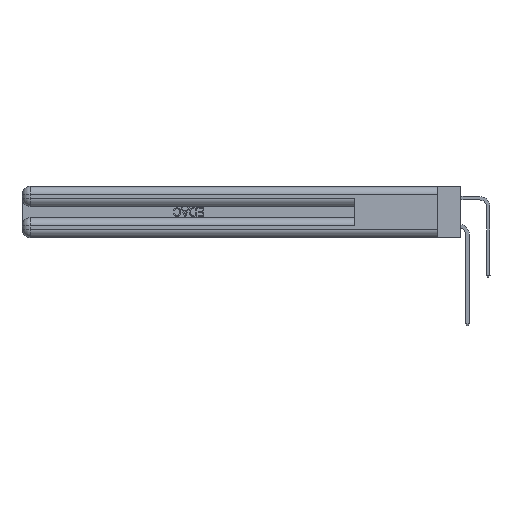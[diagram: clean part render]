
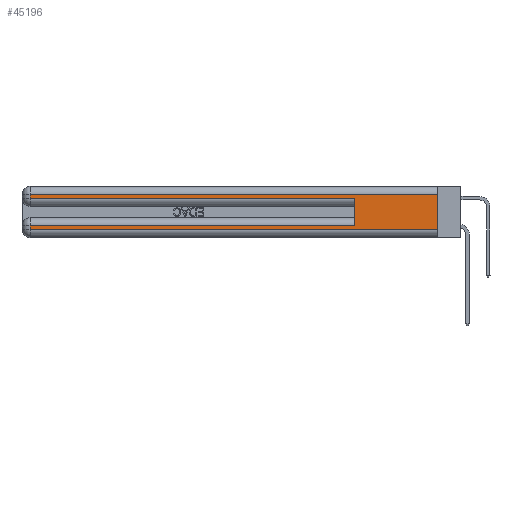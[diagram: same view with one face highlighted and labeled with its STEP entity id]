
A CAD part, left-side view. The second image highlights one B-rep face of the part: STEP entity #45196.
In plain terms, the highlighted planar face has unit normal (-1, 0, 0).
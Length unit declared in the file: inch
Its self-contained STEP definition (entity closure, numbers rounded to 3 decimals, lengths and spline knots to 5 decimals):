
#705 = DIRECTION ( 'NONE',  ( 0., 0., -1. ) ) ;
#1729 = EDGE_LOOP ( 'NONE', ( #14776, #45961, #12684, #37236, #11976, #14277, #4762, #40636 ) ) ;
#2583 = CARTESIAN_POINT ( 'NONE',  ( 0., 0., 0.06 ) ) ;
#3028 = CARTESIAN_POINT ( 'NONE',  ( 0., 0., 0.085 ) ) ;
#3943 = CARTESIAN_POINT ( 'NONE',  ( 0., 0.6, 0.145 ) ) ;
#4076 = CARTESIAN_POINT ( 'NONE',  ( 0., 0., 0.37 ) ) ;
#4349 = CARTESIAN_POINT ( 'NONE',  ( 0., 0., 0.285 ) ) ;
#4762 = ORIENTED_EDGE ( 'NONE', *, *, #11932, .T. ) ;
#5708 = EDGE_CURVE ( 'NONE', #19488, #32382, #12254, .T. ) ;
#5783 = CARTESIAN_POINT ( 'NONE',  ( 0., 0.6, 0.285 ) ) ;
#6198 = CARTESIAN_POINT ( 'NONE',  ( 0., 0.6, 0.085 ) ) ;
#6210 = VERTEX_POINT ( 'NONE', #19392 ) ;
#6652 = LINE ( 'NONE', #2583, #27688 ) ;
#6951 = CARTESIAN_POINT ( 'NONE',  ( 0., 0., 0.31 ) ) ;
#7152 = EDGE_CURVE ( 'NONE', #19488, #37345, #27515, .T. ) ;
#9133 = LINE ( 'NONE', #25689, #40958 ) ;
#9189 = CARTESIAN_POINT ( 'NONE',  ( 0., 2.94, 0.085 ) ) ;
#11681 = CARTESIAN_POINT ( 'NONE',  ( 0., 0., 0.06 ) ) ;
#11932 = EDGE_CURVE ( 'NONE', #27845, #13278, #39728, .T. ) ;
#11976 = ORIENTED_EDGE ( 'NONE', *, *, #37892, .F. ) ;
#12254 = LINE ( 'NONE', #14886, #40137 ) ;
#12684 = ORIENTED_EDGE ( 'NONE', *, *, #36053, .T. ) ;
#12790 = EDGE_CURVE ( 'NONE', #6210, #20750, #14136, .T. ) ;
#13278 = VERTEX_POINT ( 'NONE', #30140 ) ;
#14136 = LINE ( 'NONE', #4349, #43670 ) ;
#14277 = ORIENTED_EDGE ( 'NONE', *, *, #26749, .T. ) ;
#14776 = ORIENTED_EDGE ( 'NONE', *, *, #7152, .F. ) ;
#14886 = CARTESIAN_POINT ( 'NONE',  ( 0., 0., 0.31 ) ) ;
#16128 = DIRECTION ( 'NONE',  ( 0., -1., 0. ) ) ;
#17498 = DIRECTION ( 'NONE',  ( 0., 0., -1. ) ) ;
#18130 = CARTESIAN_POINT ( 'NONE',  ( 0., 2.94, 0.37 ) ) ;
#19392 = CARTESIAN_POINT ( 'NONE',  ( 0., 2.94, 0.285 ) ) ;
#19488 = VERTEX_POINT ( 'NONE', #6951 ) ;
#20701 = VECTOR ( 'NONE', #45680, 39.37008 ) ;
#20750 = VERTEX_POINT ( 'NONE', #5783 ) ;
#20902 = EDGE_CURVE ( 'NONE', #13278, #37345, #6652, .T. ) ;
#20932 = DIRECTION ( 'NONE',  ( 0., -1., 0. ) ) ;
#22026 = LINE ( 'NONE', #3028, #23170 ) ;
#23170 = VECTOR ( 'NONE', #25055, 39.37008 ) ;
#24401 = VECTOR ( 'NONE', #17498, 39.37008 ) ;
#25055 = DIRECTION ( 'NONE',  ( 0., 1., 0. ) ) ;
#25689 = CARTESIAN_POINT ( 'NONE',  ( 0., 2.94, 0.37 ) ) ;
#26053 = DIRECTION ( 'NONE',  ( 1., 0., 0. ) ) ;
#26078 = DIRECTION ( 'NONE',  ( 0., 0., 1. ) ) ;
#26749 = EDGE_CURVE ( 'NONE', #32132, #27845, #22026, .T. ) ;
#27515 = LINE ( 'NONE', #34404, #20701 ) ;
#27688 = VECTOR ( 'NONE', #20932, 39.37008 ) ;
#27845 = VERTEX_POINT ( 'NONE', #9189 ) ;
#29171 = FACE_OUTER_BOUND ( 'NONE', #1729, .T. ) ;
#29429 = PLANE ( 'NONE',  #33863 ) ;
#30140 = CARTESIAN_POINT ( 'NONE',  ( 0., 2.94, 0.06 ) ) ;
#32132 = VERTEX_POINT ( 'NONE', #6198 ) ;
#32295 = VECTOR ( 'NONE', #26078, 39.37008 ) ;
#32382 = VERTEX_POINT ( 'NONE', #43817 ) ;
#32991 = DIRECTION ( 'NONE',  ( 0., 0., -1. ) ) ;
#33863 = AXIS2_PLACEMENT_3D ( 'NONE', #4076, #26053, #705 ) ;
#34404 = CARTESIAN_POINT ( 'NONE',  ( 0., 0., 0.37 ) ) ;
#36053 = EDGE_CURVE ( 'NONE', #32382, #6210, #9133, .T. ) ;
#37236 = ORIENTED_EDGE ( 'NONE', *, *, #12790, .T. ) ;
#37345 = VERTEX_POINT ( 'NONE', #11681 ) ;
#37892 = EDGE_CURVE ( 'NONE', #32132, #20750, #44180, .T. ) ;
#39728 = LINE ( 'NONE', #18130, #24401 ) ;
#40137 = VECTOR ( 'NONE', #44726, 39.37008 ) ;
#40636 = ORIENTED_EDGE ( 'NONE', *, *, #20902, .T. ) ;
#40958 = VECTOR ( 'NONE', #32991, 39.37008 ) ;
#43670 = VECTOR ( 'NONE', #16128, 39.37008 ) ;
#43817 = CARTESIAN_POINT ( 'NONE',  ( 0., 2.94, 0.31 ) ) ;
#44180 = LINE ( 'NONE', #3943, #32295 ) ;
#44726 = DIRECTION ( 'NONE',  ( 0., 1., 0. ) ) ;
#45196 = ADVANCED_FACE ( 'NONE', ( #29171 ), #29429, .F. ) ;
#45680 = DIRECTION ( 'NONE',  ( 0., 0., -1. ) ) ;
#45961 = ORIENTED_EDGE ( 'NONE', *, *, #5708, .T. ) ;
